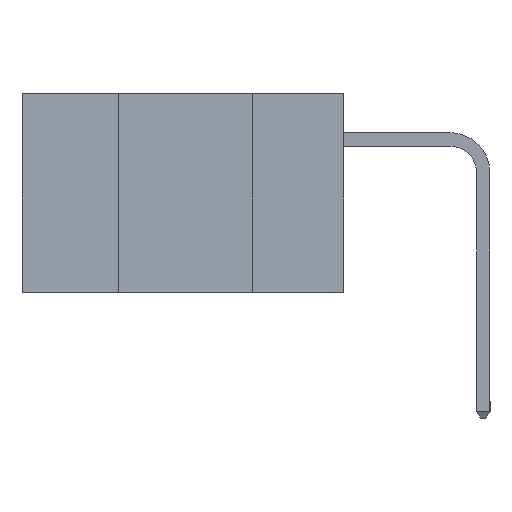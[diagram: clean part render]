
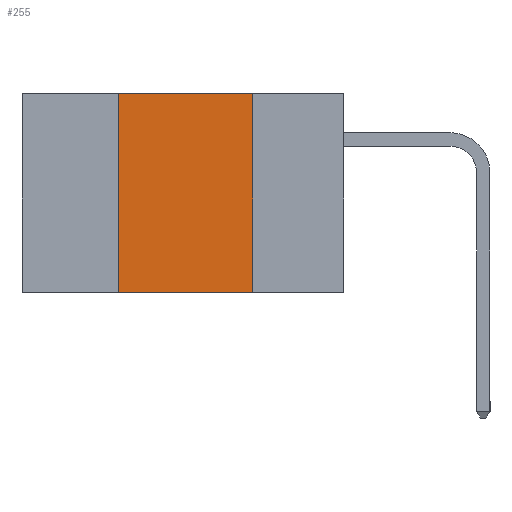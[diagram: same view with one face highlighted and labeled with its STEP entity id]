
A CAD part, left-side view. The second image highlights one B-rep face of the part: STEP entity #255.
In plain terms, the highlighted planar face has unit normal (-1, 0, 0).
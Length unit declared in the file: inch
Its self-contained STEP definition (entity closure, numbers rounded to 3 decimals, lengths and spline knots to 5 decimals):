
#139 = EDGE_CURVE ( 'NONE', #8411, #993, #928, .T. ) ;
#255 = ADVANCED_FACE ( 'NONE', ( #5671 ), #5881, .F. ) ;
#602 = CARTESIAN_POINT ( 'NONE',  ( 0., 0.42, 0. ) ) ;
#928 = LINE ( 'NONE', #1037, #5022 ) ;
#993 = VERTEX_POINT ( 'NONE', #2108 ) ;
#1037 = CARTESIAN_POINT ( 'NONE',  ( 0., 0.6, 0. ) ) ;
#1157 = CARTESIAN_POINT ( 'NONE',  ( 0., 0.6, -0.37 ) ) ;
#1983 = VERTEX_POINT ( 'NONE', #6895 ) ;
#2108 = CARTESIAN_POINT ( 'NONE',  ( 0., 0.17, 0. ) ) ;
#2128 = ORIENTED_EDGE ( 'NONE', *, *, #3130, .F. ) ;
#2338 = VECTOR ( 'NONE', #8482, 39.37008 ) ;
#2514 = VECTOR ( 'NONE', #6816, 39.37008 ) ;
#3130 = EDGE_CURVE ( 'NONE', #993, #3335, #9822, .T. ) ;
#3335 = VERTEX_POINT ( 'NONE', #10447 ) ;
#3856 = CARTESIAN_POINT ( 'NONE',  ( 0., 0.6, 0. ) ) ;
#3986 = ORIENTED_EDGE ( 'NONE', *, *, #8085, .T. ) ;
#4313 = LINE ( 'NONE', #1157, #2514 ) ;
#5022 = VECTOR ( 'NONE', #8908, 39.37008 ) ;
#5671 = FACE_OUTER_BOUND ( 'NONE', #8776, .T. ) ;
#5881 = PLANE ( 'NONE',  #5915 ) ;
#5915 = AXIS2_PLACEMENT_3D ( 'NONE', #3856, #6650, #9016 ) ;
#5937 = CARTESIAN_POINT ( 'NONE',  ( 0., 0.17, -0.37 ) ) ;
#6095 = ORIENTED_EDGE ( 'NONE', *, *, #9614, .F. ) ;
#6286 = LINE ( 'NONE', #7703, #2338 ) ;
#6561 = DIRECTION ( 'NONE',  ( 0., 0., -1. ) ) ;
#6650 = DIRECTION ( 'NONE',  ( 1., 0., 0. ) ) ;
#6816 = DIRECTION ( 'NONE',  ( 0., -1., 0. ) ) ;
#6895 = CARTESIAN_POINT ( 'NONE',  ( 0., 0.42, -0.37 ) ) ;
#7558 = VECTOR ( 'NONE', #6561, 39.37008 ) ;
#7703 = CARTESIAN_POINT ( 'NONE',  ( 0., 0.42, -0.37 ) ) ;
#8085 = EDGE_CURVE ( 'NONE', #1983, #3335, #4313, .T. ) ;
#8213 = ORIENTED_EDGE ( 'NONE', *, *, #139, .F. ) ;
#8411 = VERTEX_POINT ( 'NONE', #602 ) ;
#8482 = DIRECTION ( 'NONE',  ( 0., 0., 1. ) ) ;
#8776 = EDGE_LOOP ( 'NONE', ( #2128, #8213, #6095, #3986 ) ) ;
#8908 = DIRECTION ( 'NONE',  ( 0., -1., 0. ) ) ;
#9016 = DIRECTION ( 'NONE',  ( 0., 0., -1. ) ) ;
#9614 = EDGE_CURVE ( 'NONE', #1983, #8411, #6286, .T. ) ;
#9822 = LINE ( 'NONE', #5937, #7558 ) ;
#10447 = CARTESIAN_POINT ( 'NONE',  ( 0., 0.17, -0.37 ) ) ;
